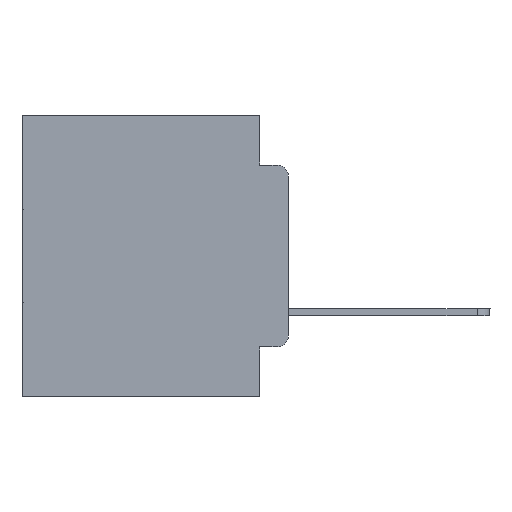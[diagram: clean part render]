
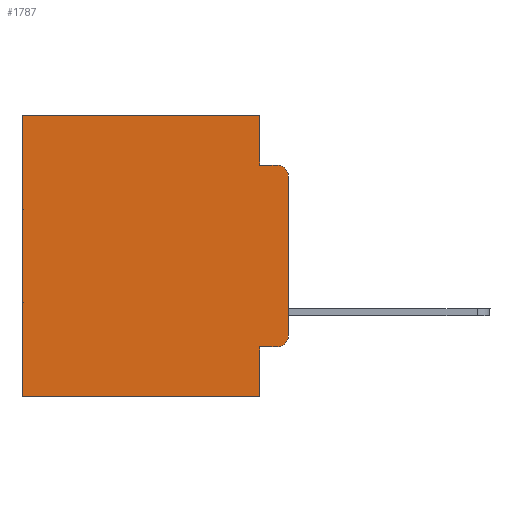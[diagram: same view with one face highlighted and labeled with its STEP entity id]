
A CAD part, left-side view. The second image highlights one B-rep face of the part: STEP entity #1787.
In plain terms, the highlighted planar face has unit normal (-1, 0, 0).
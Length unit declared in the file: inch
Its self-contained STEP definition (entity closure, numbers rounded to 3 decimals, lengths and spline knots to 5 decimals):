
#334 = ORIENTED_EDGE ( 'NONE', *, *, #22023, .F. ) ;
#428 = CARTESIAN_POINT ( 'NONE',  ( 0.298, 0.473, 0. ) ) ;
#604 = DIRECTION ( 'NONE',  ( 0., 0., -1. ) ) ;
#1021 = AXIS2_PLACEMENT_3D ( 'NONE', #20961, #2442, #21347 ) ;
#1787 = ADVANCED_FACE ( 'NONE', ( #24169 ), #13604, .F. ) ;
#1793 = VERTEX_POINT ( 'NONE', #11249 ) ;
#1893 = ORIENTED_EDGE ( 'NONE', *, *, #10230, .T. ) ;
#1895 = DIRECTION ( 'NONE',  ( -1., 0., 0. ) ) ;
#2350 = AXIS2_PLACEMENT_3D ( 'NONE', #20738, #22955, #25348 ) ;
#2442 = DIRECTION ( 'NONE',  ( -1., 0., 0. ) ) ;
#2485 = CARTESIAN_POINT ( 'NONE',  ( 0.298, 0.051, -0.0885 ) ) ;
#2854 = VERTEX_POINT ( 'NONE', #21851 ) ;
#2874 = LINE ( 'NONE', #14916, #16524 ) ;
#3683 = ORIENTED_EDGE ( 'NONE', *, *, #23140, .F. ) ;
#3737 = DIRECTION ( 'NONE',  ( 0., 0., -1. ) ) ;
#5114 = ORIENTED_EDGE ( 'NONE', *, *, #22951, .T. ) ;
#5211 = VERTEX_POINT ( 'NONE', #9126 ) ;
#5387 = VERTEX_POINT ( 'NONE', #2485 ) ;
#5906 = DIRECTION ( 'NONE',  ( 0., -1., 0. ) ) ;
#6266 = CARTESIAN_POINT ( 'NONE',  ( 0.298, 0.473, -0.5 ) ) ;
#6689 = EDGE_LOOP ( 'NONE', ( #13816, #5114, #3683, #25259, #28339, #1893, #28414, #334, #25395, #17504 ) ) ;
#7340 = CARTESIAN_POINT ( 'NONE',  ( 0.298, 0.02, -0.4115 ) ) ;
#7438 = DIRECTION ( 'NONE',  ( 0., -1., 0. ) ) ;
#7508 = DIRECTION ( 'NONE',  ( 0., 1., 0. ) ) ;
#8701 = CARTESIAN_POINT ( 'NONE',  ( 0.298, 0.051, -0.4115 ) ) ;
#9126 = CARTESIAN_POINT ( 'NONE',  ( 0.298, 0.051, 0. ) ) ;
#9130 = CARTESIAN_POINT ( 'NONE',  ( 0.298, 0.02, -0.1085 ) ) ;
#10170 = VECTOR ( 'NONE', #3737, 39.37008 ) ;
#10230 = EDGE_CURVE ( 'NONE', #1793, #15825, #20019, .T. ) ;
#10338 = DIRECTION ( 'NONE',  ( 0., 0., -1. ) ) ;
#10397 = VERTEX_POINT ( 'NONE', #12401 ) ;
#11249 = CARTESIAN_POINT ( 'NONE',  ( 0.298, 0.473, 0. ) ) ;
#11959 = VECTOR ( 'NONE', #5906, 39.37008 ) ;
#12401 = CARTESIAN_POINT ( 'NONE',  ( 0.298, 0.051, -0.4115 ) ) ;
#12557 = EDGE_CURVE ( 'NONE', #5211, #1793, #2874, .T. ) ;
#12750 = DIRECTION ( 'NONE',  ( 0., 0., -1. ) ) ;
#13604 = PLANE ( 'NONE',  #2350 ) ;
#13816 = ORIENTED_EDGE ( 'NONE', *, *, #17395, .F. ) ;
#14088 = VECTOR ( 'NONE', #10338, 39.37008 ) ;
#14411 = VECTOR ( 'NONE', #12750, 39.37008 ) ;
#14778 = CARTESIAN_POINT ( 'NONE',  ( 0.298, 0., -0.3915 ) ) ;
#14916 = CARTESIAN_POINT ( 'NONE',  ( 0.298, 0., 0. ) ) ;
#15199 = AXIS2_PLACEMENT_3D ( 'NONE', #9130, #1895, #23125 ) ;
#15825 = VERTEX_POINT ( 'NONE', #6266 ) ;
#16374 = CARTESIAN_POINT ( 'NONE',  ( 0.298, 0.02, -0.0885 ) ) ;
#16524 = VECTOR ( 'NONE', #29260, 39.37008 ) ;
#17395 = EDGE_CURVE ( 'NONE', #2854, #18342, #26826, .T. ) ;
#17504 = ORIENTED_EDGE ( 'NONE', *, *, #25615, .T. ) ;
#17925 = EDGE_CURVE ( 'NONE', #5211, #5387, #28266, .T. ) ;
#18250 = CIRCLE ( 'NONE', #1021, 0.02 ) ;
#18342 = VERTEX_POINT ( 'NONE', #14778 ) ;
#18347 = EDGE_CURVE ( 'NONE', #24582, #15825, #28608, .T. ) ;
#19673 = CARTESIAN_POINT ( 'NONE',  ( 0.298, 0., 0. ) ) ;
#19958 = CARTESIAN_POINT ( 'NONE',  ( 0.298, 0.051, -0.5 ) ) ;
#19989 = VERTEX_POINT ( 'NONE', #16374 ) ;
#20019 = LINE ( 'NONE', #428, #14088 ) ;
#20683 = CARTESIAN_POINT ( 'NONE',  ( 0.298, 0.051, 0. ) ) ;
#20738 = CARTESIAN_POINT ( 'NONE',  ( 0.298, 0., 0. ) ) ;
#20961 = CARTESIAN_POINT ( 'NONE',  ( 0.298, 0.02, -0.3915 ) ) ;
#21347 = DIRECTION ( 'NONE',  ( 0., 0., -1. ) ) ;
#21851 = CARTESIAN_POINT ( 'NONE',  ( 0.298, 0., -0.1085 ) ) ;
#22023 = EDGE_CURVE ( 'NONE', #10397, #24582, #26956, .T. ) ;
#22102 = CIRCLE ( 'NONE', #15199, 0.02 ) ;
#22812 = VECTOR ( 'NONE', #7438, 39.37008 ) ;
#22951 = EDGE_CURVE ( 'NONE', #2854, #19989, #22102, .T. ) ;
#22955 = DIRECTION ( 'NONE',  ( 1., 0., 0. ) ) ;
#23125 = DIRECTION ( 'NONE',  ( 0., 0., -1. ) ) ;
#23140 = EDGE_CURVE ( 'NONE', #5387, #19989, #24636, .T. ) ;
#23614 = CARTESIAN_POINT ( 'NONE',  ( 0.298, 0.051, -0.0885 ) ) ;
#23720 = LINE ( 'NONE', #8701, #11959 ) ;
#23800 = VECTOR ( 'NONE', #7508, 39.37008 ) ;
#24169 = FACE_OUTER_BOUND ( 'NONE', #6689, .T. ) ;
#24582 = VERTEX_POINT ( 'NONE', #19958 ) ;
#24636 = LINE ( 'NONE', #23614, #22812 ) ;
#25259 = ORIENTED_EDGE ( 'NONE', *, *, #17925, .F. ) ;
#25348 = DIRECTION ( 'NONE',  ( 0., 0., -1. ) ) ;
#25395 = ORIENTED_EDGE ( 'NONE', *, *, #26462, .T. ) ;
#25615 = EDGE_CURVE ( 'NONE', #30049, #18342, #18250, .T. ) ;
#26462 = EDGE_CURVE ( 'NONE', #10397, #30049, #23720, .T. ) ;
#26589 = CARTESIAN_POINT ( 'NONE',  ( 0.298, 0., -0.5 ) ) ;
#26826 = LINE ( 'NONE', #19673, #29045 ) ;
#26956 = LINE ( 'NONE', #28934, #14411 ) ;
#28266 = LINE ( 'NONE', #20683, #10170 ) ;
#28339 = ORIENTED_EDGE ( 'NONE', *, *, #12557, .T. ) ;
#28414 = ORIENTED_EDGE ( 'NONE', *, *, #18347, .F. ) ;
#28608 = LINE ( 'NONE', #26589, #23800 ) ;
#28934 = CARTESIAN_POINT ( 'NONE',  ( 0.298, 0.051, 0. ) ) ;
#29045 = VECTOR ( 'NONE', #604, 39.37008 ) ;
#29260 = DIRECTION ( 'NONE',  ( 0., 1., 0. ) ) ;
#30049 = VERTEX_POINT ( 'NONE', #7340 ) ;
